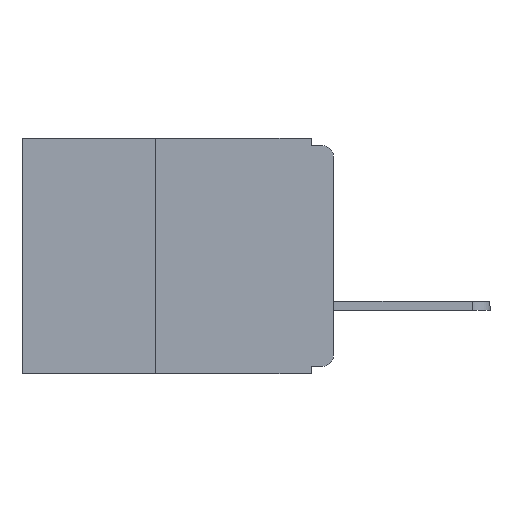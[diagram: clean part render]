
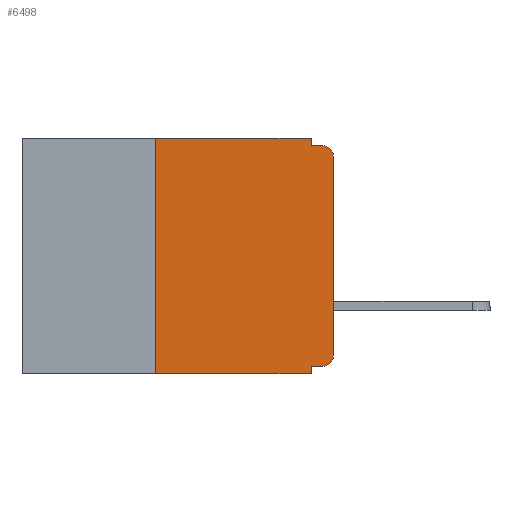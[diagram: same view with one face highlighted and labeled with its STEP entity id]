
A CAD part, left-side view. The second image highlights one B-rep face of the part: STEP entity #6498.
In plain terms, the highlighted planar face has unit normal (-1, 0, 0).
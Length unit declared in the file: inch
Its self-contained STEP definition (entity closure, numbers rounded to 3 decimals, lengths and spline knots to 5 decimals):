
#179 = DIRECTION ( 'NONE',  ( 0., 0., 1. ) ) ;
#254 = LINE ( 'NONE', #6312, #9894 ) ;
#1193 = ORIENTED_EDGE ( 'NONE', *, *, #4891, .F. ) ;
#1200 = LINE ( 'NONE', #21857, #10857 ) ;
#1414 = DIRECTION ( 'NONE',  ( -1., 0., 0. ) ) ;
#1819 = ORIENTED_EDGE ( 'NONE', *, *, #13419, .T. ) ;
#2176 = EDGE_CURVE ( 'NONE', #6980, #20996, #12720, .T. ) ;
#2510 = ORIENTED_EDGE ( 'NONE', *, *, #9506, .T. ) ;
#2933 = CARTESIAN_POINT ( 'NONE',  ( 0., 0.437, 0. ) ) ;
#3110 = LINE ( 'NONE', #5046, #7651 ) ;
#3378 = DIRECTION ( 'NONE',  ( 0., -1., 0. ) ) ;
#3506 = FACE_OUTER_BOUND ( 'NONE', #10902, .T. ) ;
#4169 = CARTESIAN_POINT ( 'NONE',  ( 0., 0.031, -0.32 ) ) ;
#4568 = CARTESIAN_POINT ( 'NONE',  ( 0., 0.25, 0. ) ) ;
#4878 = DIRECTION ( 'NONE',  ( 0., 0., -1. ) ) ;
#4891 = EDGE_CURVE ( 'NONE', #9915, #12940, #20054, .T. ) ;
#5046 = CARTESIAN_POINT ( 'NONE',  ( 0., 0.031, -0.33 ) ) ;
#5075 = CARTESIAN_POINT ( 'NONE',  ( 0., 0.031, -0.01 ) ) ;
#5399 = VERTEX_POINT ( 'NONE', #7195 ) ;
#5853 = VECTOR ( 'NONE', #179, 39.37008 ) ;
#5911 = CARTESIAN_POINT ( 'NONE',  ( 0., 0., 0. ) ) ;
#5937 = CIRCLE ( 'NONE', #21906, 0.015 ) ;
#6312 = CARTESIAN_POINT ( 'NONE',  ( 0., 0.437, 0. ) ) ;
#6371 = VERTEX_POINT ( 'NONE', #23567 ) ;
#6459 = LINE ( 'NONE', #5911, #5853 ) ;
#6498 = ADVANCED_FACE ( 'NONE', ( #3506 ), #14468, .F. ) ;
#6642 = CARTESIAN_POINT ( 'NONE',  ( 0., 0.015, -0.32 ) ) ;
#6980 = VERTEX_POINT ( 'NONE', #6642 ) ;
#6995 = DIRECTION ( 'NONE',  ( 0., 0., -1. ) ) ;
#7195 = CARTESIAN_POINT ( 'NONE',  ( 0., 0.031, 0. ) ) ;
#7211 = DIRECTION ( 'NONE',  ( -1., 0., 0. ) ) ;
#7583 = DIRECTION ( 'NONE',  ( 0., 0., -1. ) ) ;
#7622 = VECTOR ( 'NONE', #16570, 39.37008 ) ;
#7651 = VECTOR ( 'NONE', #6995, 39.37008 ) ;
#8257 = DIRECTION ( 'NONE',  ( 0., -1., 0. ) ) ;
#9506 = EDGE_CURVE ( 'NONE', #9828, #17305, #13568, .T. ) ;
#9828 = VERTEX_POINT ( 'NONE', #13756 ) ;
#9894 = VECTOR ( 'NONE', #8257, 39.37008 ) ;
#9915 = VERTEX_POINT ( 'NONE', #24040 ) ;
#10398 = CARTESIAN_POINT ( 'NONE',  ( 0., 0., -0.32 ) ) ;
#10857 = VECTOR ( 'NONE', #23756, 39.37008 ) ;
#10877 = VECTOR ( 'NONE', #7583, 39.37008 ) ;
#10902 = EDGE_LOOP ( 'NONE', ( #1819, #2510, #11391, #18594, #19790, #1193, #24257, #15288, #22200, #24586 ) ) ;
#11282 = VECTOR ( 'NONE', #3378, 39.37008 ) ;
#11391 = ORIENTED_EDGE ( 'NONE', *, *, #13196, .F. ) ;
#12720 = LINE ( 'NONE', #10398, #7622 ) ;
#12940 = VERTEX_POINT ( 'NONE', #4568 ) ;
#12953 = CARTESIAN_POINT ( 'NONE',  ( 0., 0.015, -0.025 ) ) ;
#13071 = CARTESIAN_POINT ( 'NONE',  ( 0., 0.25, -0.33 ) ) ;
#13175 = DIRECTION ( 'NONE',  ( 0., 0., 1. ) ) ;
#13196 = EDGE_CURVE ( 'NONE', #20198, #17305, #21463, .T. ) ;
#13419 = EDGE_CURVE ( 'NONE', #6371, #9828, #6459, .T. ) ;
#13568 = CIRCLE ( 'NONE', #19988, 0.015 ) ;
#13756 = CARTESIAN_POINT ( 'NONE',  ( 0., 0., -0.025 ) ) ;
#13784 = EDGE_CURVE ( 'NONE', #20996, #23613, #3110, .T. ) ;
#14468 = PLANE ( 'NONE',  #16730 ) ;
#14874 = DIRECTION ( 'NONE',  ( 0., 0., -1. ) ) ;
#14900 = CARTESIAN_POINT ( 'NONE',  ( 0., 0., -0.01 ) ) ;
#14991 = VECTOR ( 'NONE', #13175, 39.37008 ) ;
#15133 = EDGE_CURVE ( 'NONE', #5399, #20198, #15946, .T. ) ;
#15288 = ORIENTED_EDGE ( 'NONE', *, *, #13784, .F. ) ;
#15946 = LINE ( 'NONE', #20948, #10877 ) ;
#16369 = DIRECTION ( 'NONE',  ( 1., 0., 0. ) ) ;
#16570 = DIRECTION ( 'NONE',  ( 0., 1., 0. ) ) ;
#16730 = AXIS2_PLACEMENT_3D ( 'NONE', #2933, #16369, #4878 ) ;
#17305 = VERTEX_POINT ( 'NONE', #19912 ) ;
#18341 = EDGE_CURVE ( 'NONE', #6980, #6371, #5937, .T. ) ;
#18594 = ORIENTED_EDGE ( 'NONE', *, *, #15133, .F. ) ;
#18642 = CARTESIAN_POINT ( 'NONE',  ( 0., 0.015, -0.305 ) ) ;
#19790 = ORIENTED_EDGE ( 'NONE', *, *, #22876, .F. ) ;
#19912 = CARTESIAN_POINT ( 'NONE',  ( 0., 0.015, -0.01 ) ) ;
#19988 = AXIS2_PLACEMENT_3D ( 'NONE', #12953, #1414, #14874 ) ;
#20054 = LINE ( 'NONE', #13071, #14991 ) ;
#20198 = VERTEX_POINT ( 'NONE', #5075 ) ;
#20579 = DIRECTION ( 'NONE',  ( 0., 0., -1. ) ) ;
#20948 = CARTESIAN_POINT ( 'NONE',  ( 0., 0.031, 0. ) ) ;
#20996 = VERTEX_POINT ( 'NONE', #4169 ) ;
#21463 = LINE ( 'NONE', #14900, #11282 ) ;
#21792 = EDGE_CURVE ( 'NONE', #9915, #23613, #1200, .T. ) ;
#21857 = CARTESIAN_POINT ( 'NONE',  ( 0., 0.437, -0.33 ) ) ;
#21906 = AXIS2_PLACEMENT_3D ( 'NONE', #18642, #7211, #20579 ) ;
#22200 = ORIENTED_EDGE ( 'NONE', *, *, #2176, .F. ) ;
#22876 = EDGE_CURVE ( 'NONE', #12940, #5399, #254, .T. ) ;
#23175 = CARTESIAN_POINT ( 'NONE',  ( 0., 0.031, -0.33 ) ) ;
#23567 = CARTESIAN_POINT ( 'NONE',  ( 0., 0., -0.305 ) ) ;
#23613 = VERTEX_POINT ( 'NONE', #23175 ) ;
#23756 = DIRECTION ( 'NONE',  ( 0., -1., 0. ) ) ;
#24040 = CARTESIAN_POINT ( 'NONE',  ( 0., 0.25, -0.33 ) ) ;
#24257 = ORIENTED_EDGE ( 'NONE', *, *, #21792, .T. ) ;
#24586 = ORIENTED_EDGE ( 'NONE', *, *, #18341, .T. ) ;
